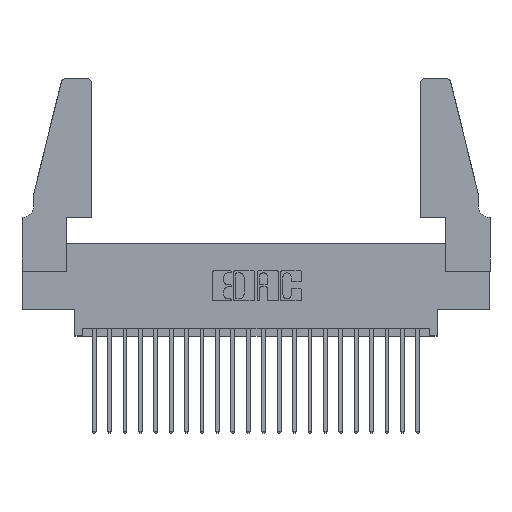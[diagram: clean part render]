
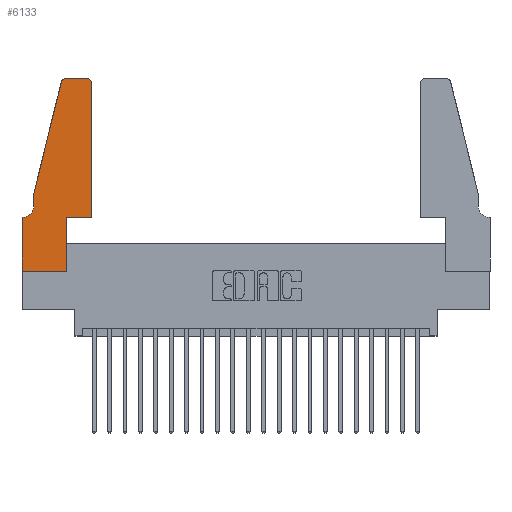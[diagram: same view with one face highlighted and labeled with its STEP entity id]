
A CAD part, top view. The second image highlights one B-rep face of the part: STEP entity #6133.
In plain terms, the highlighted planar face has unit normal (0, 0, 1).
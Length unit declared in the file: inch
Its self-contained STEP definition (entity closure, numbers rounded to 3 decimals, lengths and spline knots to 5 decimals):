
#176 = EDGE_LOOP ( 'NONE', ( #2682, #15193, #21537, #15271, #20042, #18218, #9727, #4686, #11217, #15456, #3514, #18495 ) ) ;
#181 = LINE ( 'NONE', #1156, #17962 ) ;
#478 = VECTOR ( 'NONE', #13657, 39.37008 ) ;
#551 = LINE ( 'NONE', #12428, #15105 ) ;
#557 = VECTOR ( 'NONE', #16790, 39.37008 ) ;
#833 = DIRECTION ( 'NONE',  ( 0., 0., -1. ) ) ;
#1156 = CARTESIAN_POINT ( 'NONE',  ( 0.0755, 0.5, 0.37 ) ) ;
#1293 = CARTESIAN_POINT ( 'NONE',  ( 0.2865, 0.35, 0.37 ) ) ;
#1307 = LINE ( 'NONE', #11937, #21483 ) ;
#1341 = CARTESIAN_POINT ( 'NONE',  ( 0.4505, 0.35, 0.37 ) ) ;
#1584 = CARTESIAN_POINT ( 'NONE',  ( 0.4505, 0.35, 0.37 ) ) ;
#1650 = CARTESIAN_POINT ( 'NONE',  ( 0.0755, 0.5, 0.37 ) ) ;
#2261 = EDGE_CURVE ( 'NONE', #16097, #4099, #7740, .T. ) ;
#2524 = AXIS2_PLACEMENT_3D ( 'NONE', #7731, #14696, #7805 ) ;
#2574 = DIRECTION ( 'NONE',  ( -1., 0., 0. ) ) ;
#2682 = ORIENTED_EDGE ( 'NONE', *, *, #2827, .T. ) ;
#2827 = EDGE_CURVE ( 'NONE', #18424, #19262, #18056, .T. ) ;
#2949 = CARTESIAN_POINT ( 'NONE',  ( 0.4205, 1.25, 0.37 ) ) ;
#3298 = CARTESIAN_POINT ( 'NONE',  ( 0., 0.35, 0.37 ) ) ;
#3509 = DIRECTION ( 'NONE',  ( 0., 1., 0. ) ) ;
#3514 = ORIENTED_EDGE ( 'NONE', *, *, #7030, .T. ) ;
#3823 = VERTEX_POINT ( 'NONE', #20424 ) ;
#3914 = CARTESIAN_POINT ( 'NONE',  ( 0.25487, 1.22718, 0.37 ) ) ;
#4099 = VERTEX_POINT ( 'NONE', #9317 ) ;
#4283 = VERTEX_POINT ( 'NONE', #1650 ) ;
#4517 = CARTESIAN_POINT ( 'NONE',  ( 0.0055, 0.42, 0.37 ) ) ;
#4600 = CARTESIAN_POINT ( 'NONE',  ( 0.2865, 0.35, 0.37 ) ) ;
#4686 = ORIENTED_EDGE ( 'NONE', *, *, #16182, .T. ) ;
#4697 = AXIS2_PLACEMENT_3D ( 'NONE', #4517, #833, #2574 ) ;
#4873 = DIRECTION ( 'NONE',  ( 1., 0., 0. ) ) ;
#5057 = DIRECTION ( 'NONE',  ( 1., 0., 0. ) ) ;
#5343 = EDGE_CURVE ( 'NONE', #21557, #17754, #21752, .T. ) ;
#5383 = DIRECTION ( 'NONE',  ( 0., 0., 1. ) ) ;
#5497 = CIRCLE ( 'NONE', #12194, 0.03 ) ;
#5653 = DIRECTION ( 'NONE',  ( 0., -1., 0. ) ) ;
#5785 = AXIS2_PLACEMENT_3D ( 'NONE', #12257, #14033, #8830 ) ;
#6044 = CARTESIAN_POINT ( 'NONE',  ( 0.4505, 0.35, 0.37 ) ) ;
#6133 = ADVANCED_FACE ( 'NONE', ( #7417 ), #13823, .T. ) ;
#7030 = EDGE_CURVE ( 'NONE', #7822, #20826, #18150, .T. ) ;
#7417 = FACE_OUTER_BOUND ( 'NONE', #176, .T. ) ;
#7495 = CARTESIAN_POINT ( 'NONE',  ( 0.0755, 0.42, 0.37 ) ) ;
#7541 = VERTEX_POINT ( 'NONE', #7495 ) ;
#7731 = CARTESIAN_POINT ( 'NONE',  ( 0.4205, 1.22, 0.37 ) ) ;
#7740 = LINE ( 'NONE', #18580, #478 ) ;
#7805 = DIRECTION ( 'NONE',  ( 1., 0., 0. ) ) ;
#7822 = VERTEX_POINT ( 'NONE', #6044 ) ;
#8417 = EDGE_CURVE ( 'NONE', #20826, #18424, #18917, .T. ) ;
#8613 = VERTEX_POINT ( 'NONE', #3914 ) ;
#8777 = EDGE_CURVE ( 'NONE', #7541, #3823, #14771, .T. ) ;
#8830 = DIRECTION ( 'NONE',  ( 1., 0., 0. ) ) ;
#9305 = DIRECTION ( 'NONE',  ( -1., 0., 0. ) ) ;
#9317 = CARTESIAN_POINT ( 'NONE',  ( 0., 0., 0.37 ) ) ;
#9701 = DIRECTION ( 'NONE',  ( -0.239, -0.971, 0. ) ) ;
#9727 = ORIENTED_EDGE ( 'NONE', *, *, #2261, .T. ) ;
#10126 = CARTESIAN_POINT ( 'NONE',  ( 0.2865, 0., 0.37 ) ) ;
#10178 = EDGE_CURVE ( 'NONE', #3823, #16097, #551, .T. ) ;
#10598 = DIRECTION ( 'NONE',  ( 1., 0., 0. ) ) ;
#10952 = LINE ( 'NONE', #14271, #11507 ) ;
#11217 = ORIENTED_EDGE ( 'NONE', *, *, #5343, .T. ) ;
#11507 = VECTOR ( 'NONE', #5653, 39.37008 ) ;
#11937 = CARTESIAN_POINT ( 'NONE',  ( 0., 0., 0.37 ) ) ;
#12194 = AXIS2_PLACEMENT_3D ( 'NONE', #15718, #5383, #10598 ) ;
#12257 = CARTESIAN_POINT ( 'NONE',  ( 0., 0.35, 0.37 ) ) ;
#12428 = CARTESIAN_POINT ( 'NONE',  ( 0.0755, 0.35, 0.37 ) ) ;
#12621 = EDGE_CURVE ( 'NONE', #8613, #4283, #181, .T. ) ;
#12771 = VECTOR ( 'NONE', #3509, 39.37008 ) ;
#13051 = EDGE_CURVE ( 'NONE', #4283, #7541, #10952, .T. ) ;
#13388 = CARTESIAN_POINT ( 'NONE',  ( 0.2605, 1.25, 0.37 ) ) ;
#13657 = DIRECTION ( 'NONE',  ( 0., -1., 0. ) ) ;
#13823 = PLANE ( 'NONE',  #5785 ) ;
#14033 = DIRECTION ( 'NONE',  ( 0., 0., 1. ) ) ;
#14271 = CARTESIAN_POINT ( 'NONE',  ( 0.0755, 0.5, 0.37 ) ) ;
#14696 = DIRECTION ( 'NONE',  ( 0., 0., 1. ) ) ;
#14707 = CARTESIAN_POINT ( 'NONE',  ( 0.4505, 1.22, 0.37 ) ) ;
#14771 = CIRCLE ( 'NONE', #4697, 0.07 ) ;
#15105 = VECTOR ( 'NONE', #9305, 39.37008 ) ;
#15193 = ORIENTED_EDGE ( 'NONE', *, *, #17965, .T. ) ;
#15271 = ORIENTED_EDGE ( 'NONE', *, *, #13051, .T. ) ;
#15280 = CARTESIAN_POINT ( 'NONE',  ( 0.284, 1.25, 0.37 ) ) ;
#15456 = ORIENTED_EDGE ( 'NONE', *, *, #16988, .T. ) ;
#15718 = CARTESIAN_POINT ( 'NONE',  ( 0.284, 1.22, 0.37 ) ) ;
#15811 = VECTOR ( 'NONE', #4873, 39.37008 ) ;
#16097 = VERTEX_POINT ( 'NONE', #3298 ) ;
#16182 = EDGE_CURVE ( 'NONE', #4099, #21557, #1307, .T. ) ;
#16790 = DIRECTION ( 'NONE',  ( -1., 0., 0. ) ) ;
#16988 = EDGE_CURVE ( 'NONE', #17754, #7822, #20390, .T. ) ;
#17181 = VECTOR ( 'NONE', #18382, 39.37008 ) ;
#17754 = VERTEX_POINT ( 'NONE', #1293 ) ;
#17962 = VECTOR ( 'NONE', #9701, 39.37008 ) ;
#17965 = EDGE_CURVE ( 'NONE', #19262, #8613, #5497, .T. ) ;
#18056 = LINE ( 'NONE', #13388, #557 ) ;
#18150 = LINE ( 'NONE', #1584, #12771 ) ;
#18218 = ORIENTED_EDGE ( 'NONE', *, *, #10178, .T. ) ;
#18382 = DIRECTION ( 'NONE',  ( 0., 1., 0. ) ) ;
#18424 = VERTEX_POINT ( 'NONE', #2949 ) ;
#18495 = ORIENTED_EDGE ( 'NONE', *, *, #8417, .T. ) ;
#18580 = CARTESIAN_POINT ( 'NONE',  ( 0., 0., 0.37 ) ) ;
#18917 = CIRCLE ( 'NONE', #2524, 0.03 ) ;
#19262 = VERTEX_POINT ( 'NONE', #15280 ) ;
#20042 = ORIENTED_EDGE ( 'NONE', *, *, #8777, .T. ) ;
#20390 = LINE ( 'NONE', #1341, #15811 ) ;
#20424 = CARTESIAN_POINT ( 'NONE',  ( 0.0055, 0.35, 0.37 ) ) ;
#20826 = VERTEX_POINT ( 'NONE', #14707 ) ;
#21483 = VECTOR ( 'NONE', #5057, 39.37008 ) ;
#21537 = ORIENTED_EDGE ( 'NONE', *, *, #12621, .T. ) ;
#21557 = VERTEX_POINT ( 'NONE', #10126 ) ;
#21752 = LINE ( 'NONE', #4600, #17181 ) ;
